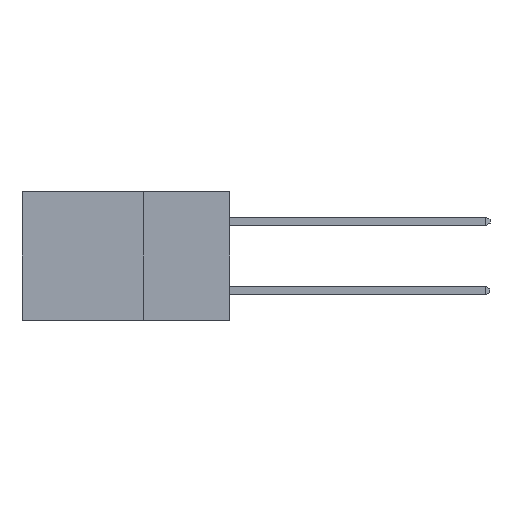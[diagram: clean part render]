
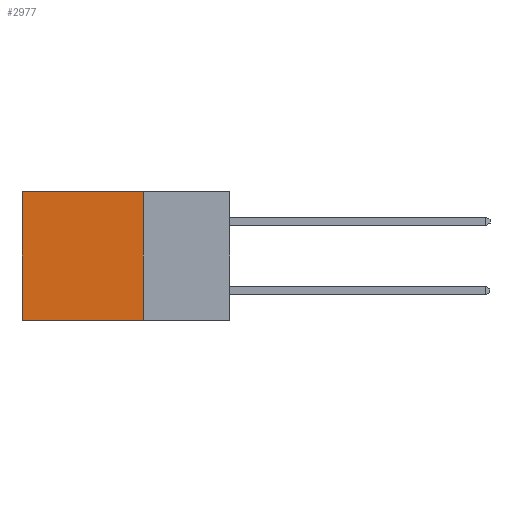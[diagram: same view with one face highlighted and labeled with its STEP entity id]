
A CAD part, left-side view. The second image highlights one B-rep face of the part: STEP entity #2977.
In plain terms, the highlighted planar face has unit normal (-1, 0, 0).
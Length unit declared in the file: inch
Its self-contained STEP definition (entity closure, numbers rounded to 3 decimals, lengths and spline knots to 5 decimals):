
#172 = LINE ( 'NONE', #1067, #12820 ) ;
#359 = EDGE_LOOP ( 'NONE', ( #12312, #3947, #12417, #3475 ) ) ;
#946 = CARTESIAN_POINT ( 'NONE',  ( 0.298, 0.25, 0. ) ) ;
#1024 = DIRECTION ( 'NONE',  ( 0., 0., -1. ) ) ;
#1067 = CARTESIAN_POINT ( 'NONE',  ( 0.298, 0.6, 0. ) ) ;
#1190 = FACE_OUTER_BOUND ( 'NONE', #359, .T. ) ;
#1269 = VERTEX_POINT ( 'NONE', #8048 ) ;
#1358 = VERTEX_POINT ( 'NONE', #14306 ) ;
#1826 = DIRECTION ( 'NONE',  ( 1., 0., 0. ) ) ;
#1838 = PLANE ( 'NONE',  #11240 ) ;
#2215 = DIRECTION ( 'NONE',  ( 0., 0., -1. ) ) ;
#2357 = CARTESIAN_POINT ( 'NONE',  ( 0.298, 0.6, 0. ) ) ;
#2977 = ADVANCED_FACE ( 'NONE', ( #1190 ), #1838, .F. ) ;
#2980 = LINE ( 'NONE', #9546, #6285 ) ;
#3267 = CARTESIAN_POINT ( 'NONE',  ( 0.298, 0.25, -0.37 ) ) ;
#3276 = EDGE_CURVE ( 'NONE', #6955, #1269, #172, .T. ) ;
#3310 = DIRECTION ( 'NONE',  ( 0., 1., 0. ) ) ;
#3475 = ORIENTED_EDGE ( 'NONE', *, *, #5602, .T. ) ;
#3567 = LINE ( 'NONE', #3267, #6089 ) ;
#3670 = VECTOR ( 'NONE', #1024, 39.37008 ) ;
#3947 = ORIENTED_EDGE ( 'NONE', *, *, #13765, .F. ) ;
#4147 = CARTESIAN_POINT ( 'NONE',  ( 0.298, 0.25, -0.37 ) ) ;
#5602 = EDGE_CURVE ( 'NONE', #1358, #6955, #2980, .T. ) ;
#6089 = VECTOR ( 'NONE', #3310, 39.37008 ) ;
#6285 = VECTOR ( 'NONE', #14811, 39.37008 ) ;
#6955 = VERTEX_POINT ( 'NONE', #2357 ) ;
#8048 = CARTESIAN_POINT ( 'NONE',  ( 0.298, 0.6, -0.37 ) ) ;
#9546 = CARTESIAN_POINT ( 'NONE',  ( 0.298, 0.25, 0. ) ) ;
#10115 = EDGE_CURVE ( 'NONE', #1358, #10551, #10165, .T. ) ;
#10165 = LINE ( 'NONE', #946, #3670 ) ;
#10551 = VERTEX_POINT ( 'NONE', #4147 ) ;
#11240 = AXIS2_PLACEMENT_3D ( 'NONE', #13489, #1826, #2215 ) ;
#12312 = ORIENTED_EDGE ( 'NONE', *, *, #3276, .T. ) ;
#12417 = ORIENTED_EDGE ( 'NONE', *, *, #10115, .F. ) ;
#12820 = VECTOR ( 'NONE', #14615, 39.37008 ) ;
#13489 = CARTESIAN_POINT ( 'NONE',  ( 0.298, 0.25, 0. ) ) ;
#13765 = EDGE_CURVE ( 'NONE', #10551, #1269, #3567, .T. ) ;
#14306 = CARTESIAN_POINT ( 'NONE',  ( 0.298, 0.25, 0. ) ) ;
#14615 = DIRECTION ( 'NONE',  ( 0., 0., -1. ) ) ;
#14811 = DIRECTION ( 'NONE',  ( 0., 1., 0. ) ) ;
